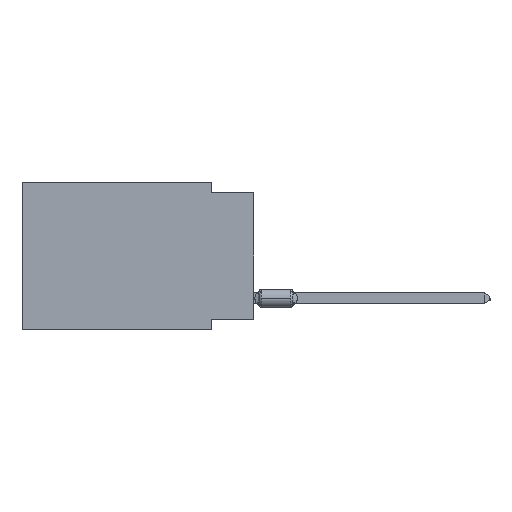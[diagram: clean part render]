
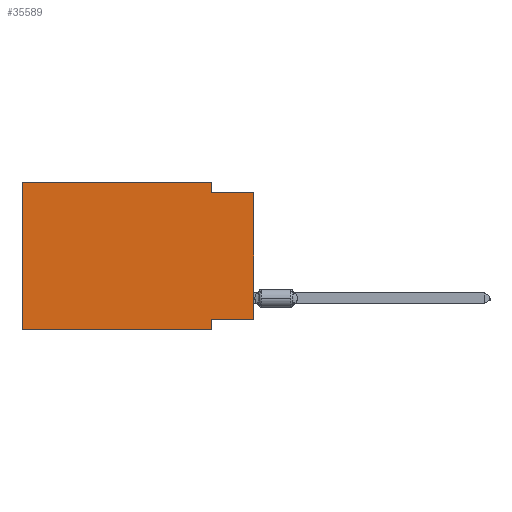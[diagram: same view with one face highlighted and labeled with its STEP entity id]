
A CAD part, left-side view. The second image highlights one B-rep face of the part: STEP entity #35589.
In plain terms, the highlighted planar face has unit normal (-1, 0, 0).
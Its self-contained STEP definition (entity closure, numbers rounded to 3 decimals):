
#190 = ORIENTED_EDGE ( 'NONE', *, *, #21428, .F. ) ;
#2285 = DIRECTION ( 'NONE',  ( 0., 0., -1. ) ) ;
#2600 = VECTOR ( 'NONE', #40011, 1000. ) ;
#3792 = ORIENTED_EDGE ( 'NONE', *, *, #13628, .F. ) ;
#3929 = LINE ( 'NONE', #46938, #33698 ) ;
#4034 = PLANE ( 'NONE',  #7692 ) ;
#4233 = CARTESIAN_POINT ( 'NONE',  ( 0., 2.54, 0. ) ) ;
#6235 = DIRECTION ( 'NONE',  ( 0., -1., 0. ) ) ;
#6544 = CARTESIAN_POINT ( 'NONE',  ( 0., 13.97, -8.89 ) ) ;
#7692 = AXIS2_PLACEMENT_3D ( 'NONE', #9291, #57862, #63112 ) ;
#8884 = VERTEX_POINT ( 'NONE', #40255 ) ;
#8895 = LINE ( 'NONE', #45616, #2600 ) ;
#9291 = CARTESIAN_POINT ( 'NONE',  ( 0., 13.97, 0. ) ) ;
#9332 = LINE ( 'NONE', #30995, #15665 ) ;
#9773 = EDGE_CURVE ( 'NONE', #14706, #67375, #9332, .T. ) ;
#10832 = LINE ( 'NONE', #43668, #12592 ) ;
#11133 = EDGE_CURVE ( 'NONE', #35375, #49689, #43638, .T. ) ;
#11523 = VERTEX_POINT ( 'NONE', #31589 ) ;
#12592 = VECTOR ( 'NONE', #68831, 1000. ) ;
#12795 = LINE ( 'NONE', #55427, #54178 ) ;
#13628 = EDGE_CURVE ( 'NONE', #62770, #62739, #55573, .T. ) ;
#14290 = CARTESIAN_POINT ( 'NONE',  ( 0., 2.54, -0.635 ) ) ;
#14706 = VERTEX_POINT ( 'NONE', #4233 ) ;
#15665 = VECTOR ( 'NONE', #26099, 1000. ) ;
#21428 = EDGE_CURVE ( 'NONE', #67375, #11523, #66815, .T. ) ;
#22281 = ORIENTED_EDGE ( 'NONE', *, *, #52112, .F. ) ;
#24012 = CARTESIAN_POINT ( 'NONE',  ( 0., 2.54, -8.89 ) ) ;
#25597 = DIRECTION ( 'NONE',  ( 0., -1., 0. ) ) ;
#26099 = DIRECTION ( 'NONE',  ( 0., 0., -1. ) ) ;
#29767 = CARTESIAN_POINT ( 'NONE',  ( 0., 0., -0.635 ) ) ;
#29897 = FACE_OUTER_BOUND ( 'NONE', #43204, .T. ) ;
#30995 = CARTESIAN_POINT ( 'NONE',  ( 0., 2.54, 0. ) ) ;
#31589 = CARTESIAN_POINT ( 'NONE',  ( 0., 0., -0.635 ) ) ;
#33698 = VECTOR ( 'NONE', #25597, 1000. ) ;
#35375 = VERTEX_POINT ( 'NONE', #6544 ) ;
#35589 = ADVANCED_FACE ( 'NONE', ( #29897 ), #4034, .F. ) ;
#35609 = CARTESIAN_POINT ( 'NONE',  ( 0., 0., -8.255 ) ) ;
#36066 = EDGE_CURVE ( 'NONE', #62739, #49689, #12795, .T. ) ;
#36367 = VECTOR ( 'NONE', #40170, 1000. ) ;
#39150 = EDGE_CURVE ( 'NONE', #8884, #14706, #3929, .T. ) ;
#39346 = VECTOR ( 'NONE', #51106, 1000. ) ;
#40011 = DIRECTION ( 'NONE',  ( 0., 0., 1. ) ) ;
#40170 = DIRECTION ( 'NONE',  ( 0., 1., 0. ) ) ;
#40255 = CARTESIAN_POINT ( 'NONE',  ( 0., 13.97, 0. ) ) ;
#43204 = EDGE_LOOP ( 'NONE', ( #51461, #190, #50656, #62597, #22281, #48958, #59394, #3792 ) ) ;
#43638 = LINE ( 'NONE', #54127, #45035 ) ;
#43668 = CARTESIAN_POINT ( 'NONE',  ( 0., 13.97, 0. ) ) ;
#45035 = VECTOR ( 'NONE', #6235, 1000. ) ;
#45433 = CARTESIAN_POINT ( 'NONE',  ( 0., 0., -8.255 ) ) ;
#45616 = CARTESIAN_POINT ( 'NONE',  ( 0., 0., 0. ) ) ;
#46938 = CARTESIAN_POINT ( 'NONE',  ( 0., 13.97, 0. ) ) ;
#48958 = ORIENTED_EDGE ( 'NONE', *, *, #11133, .T. ) ;
#49689 = VERTEX_POINT ( 'NONE', #24012 ) ;
#50656 = ORIENTED_EDGE ( 'NONE', *, *, #9773, .F. ) ;
#51036 = CARTESIAN_POINT ( 'NONE',  ( 0., 2.54, -8.255 ) ) ;
#51106 = DIRECTION ( 'NONE',  ( 0., -1., 0. ) ) ;
#51461 = ORIENTED_EDGE ( 'NONE', *, *, #61904, .T. ) ;
#52112 = EDGE_CURVE ( 'NONE', #35375, #8884, #10832, .T. ) ;
#54127 = CARTESIAN_POINT ( 'NONE',  ( 0., 13.97, -8.89 ) ) ;
#54178 = VECTOR ( 'NONE', #2285, 1000. ) ;
#55427 = CARTESIAN_POINT ( 'NONE',  ( 0., 2.54, -8.89 ) ) ;
#55573 = LINE ( 'NONE', #45433, #36367 ) ;
#57862 = DIRECTION ( 'NONE',  ( 1., 0., 0. ) ) ;
#59394 = ORIENTED_EDGE ( 'NONE', *, *, #36066, .F. ) ;
#61904 = EDGE_CURVE ( 'NONE', #62770, #11523, #8895, .T. ) ;
#62597 = ORIENTED_EDGE ( 'NONE', *, *, #39150, .F. ) ;
#62739 = VERTEX_POINT ( 'NONE', #51036 ) ;
#62770 = VERTEX_POINT ( 'NONE', #35609 ) ;
#63112 = DIRECTION ( 'NONE',  ( 0., 0., -1. ) ) ;
#66815 = LINE ( 'NONE', #29767, #39346 ) ;
#67375 = VERTEX_POINT ( 'NONE', #14290 ) ;
#68831 = DIRECTION ( 'NONE',  ( 0., 0., 1. ) ) ;
